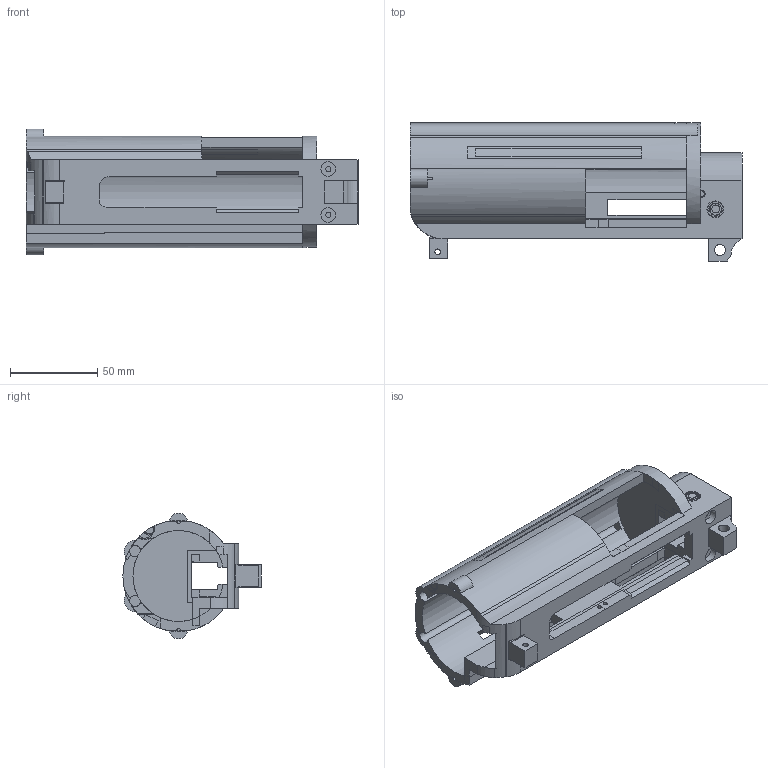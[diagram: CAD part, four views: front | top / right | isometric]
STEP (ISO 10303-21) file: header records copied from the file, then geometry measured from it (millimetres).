
FILE_DESCRIPTION(('FreeCAD Model'),'2;1');
FILE_NAME('mp-1 upper (gluty ready).step','2016-03-27T02:49:51',('Author'),(''), 'Open CASCADE STEP processor 6.8','FreeCAD','Unknown');
FILE_SCHEMA(('AUTOMOTIVE_DESIGN_CC2 { 1 2 10303 214 -1 1 5 4 }'));
Length unit declared in the file: millimetre
Products named in the file (1): Pocket045
Bounding box: 190.5 x 79.31 x 72.04 mm (x, y, z)
Volume: 210976 mm3; surface area: 79679.9 mm2
Topology: 1 solids, 1 shells, 311 faces, 922 edges, 614 vertices
Faces by surface type: plane 254, cylinder 57
Full cylindrical faces by diameter (mm): 2 x4, 2.4 x6, 8 x1, 8.4 x2
Entity records: 23712 total; most frequent: CARTESIAN_POINT 6786, DIRECTION 2809, ORIENTED_EDGE 1844, PCURVE 1844, DEFINITIONAL_REPRESENTATION 1844, LINE 1580, VECTOR 1580, EDGE_CURVE 922
